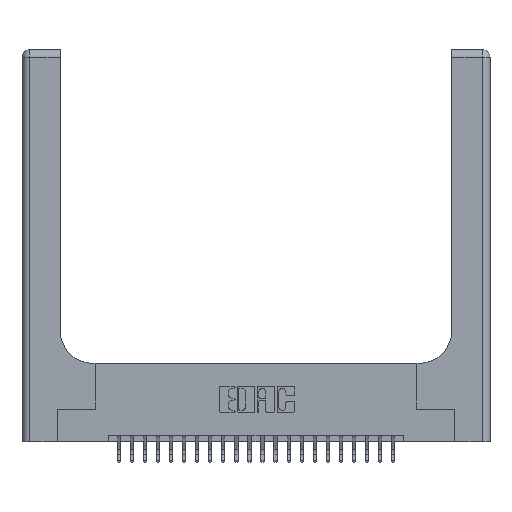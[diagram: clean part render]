
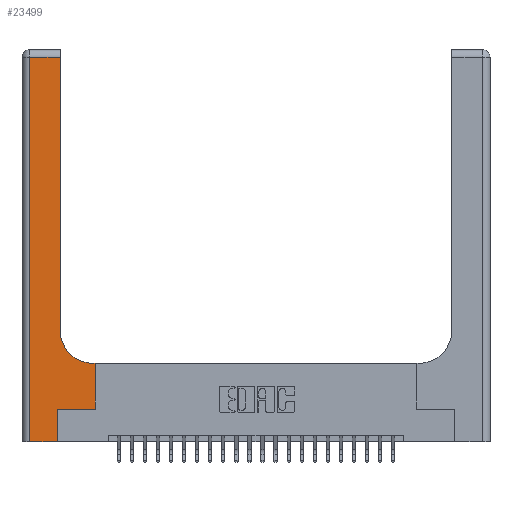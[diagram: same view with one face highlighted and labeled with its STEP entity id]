
A CAD part, top view. The second image highlights one B-rep face of the part: STEP entity #23499.
In plain terms, the highlighted planar face has unit normal (0, 0, 1).
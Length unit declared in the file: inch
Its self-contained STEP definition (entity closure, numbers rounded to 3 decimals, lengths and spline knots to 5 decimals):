
#33 = CARTESIAN_POINT ( 'NONE',  ( 0., 0., 0.37 ) ) ;
#120 = VECTOR ( 'NONE', #15755, 39.37008 ) ;
#164 = DIRECTION ( 'NONE',  ( 0., 1., 0. ) ) ;
#365 = LINE ( 'NONE', #9167, #15659 ) ;
#517 = CARTESIAN_POINT ( 'NONE',  ( 0.2915, 3., 0.37 ) ) ;
#683 = VERTEX_POINT ( 'NONE', #3446 ) ;
#2593 = EDGE_CURVE ( 'NONE', #6802, #8842, #365, .T. ) ;
#2601 = LINE ( 'NONE', #12190, #13845 ) ;
#2632 = EDGE_CURVE ( 'NONE', #4850, #683, #25175, .T. ) ;
#2824 = CARTESIAN_POINT ( 'NONE',  ( 0.269, 0., 0.37 ) ) ;
#3270 = DIRECTION ( 'NONE',  ( 0., 1., 0. ) ) ;
#3446 = CARTESIAN_POINT ( 'NONE',  ( 0.2915, 0.85, 0.37 ) ) ;
#4015 = ORIENTED_EDGE ( 'NONE', *, *, #16800, .T. ) ;
#4016 = EDGE_LOOP ( 'NONE', ( #20189, #21307, #7704, #24656, #18710, #25285, #23282, #4015, #7865 ) ) ;
#4236 = CARTESIAN_POINT ( 'NONE',  ( 0.269, 0.25, 0.37 ) ) ;
#4583 = DIRECTION ( 'NONE',  ( 0., 1., 0. ) ) ;
#4655 = LINE ( 'NONE', #24790, #24748 ) ;
#4850 = VERTEX_POINT ( 'NONE', #16974 ) ;
#5414 = VERTEX_POINT ( 'NONE', #6796 ) ;
#5592 = VERTEX_POINT ( 'NONE', #19182 ) ;
#5968 = EDGE_CURVE ( 'NONE', #683, #18829, #17972, .T. ) ;
#6436 = VECTOR ( 'NONE', #21737, 39.37008 ) ;
#6667 = VERTEX_POINT ( 'NONE', #16339 ) ;
#6796 = CARTESIAN_POINT ( 'NONE',  ( 0.06, 2.94, 0.37 ) ) ;
#6802 = VERTEX_POINT ( 'NONE', #2824 ) ;
#6946 = VECTOR ( 'NONE', #8156, 39.37008 ) ;
#7271 = CARTESIAN_POINT ( 'NONE',  ( 0.06, 3., 0.37 ) ) ;
#7704 = ORIENTED_EDGE ( 'NONE', *, *, #23745, .T. ) ;
#7865 = ORIENTED_EDGE ( 'NONE', *, *, #2632, .T. ) ;
#8156 = DIRECTION ( 'NONE',  ( 1., 0., 0. ) ) ;
#8186 = VECTOR ( 'NONE', #4583, 39.37008 ) ;
#8596 = DIRECTION ( 'NONE',  ( 0., 0., -1. ) ) ;
#8842 = VERTEX_POINT ( 'NONE', #4236 ) ;
#9167 = CARTESIAN_POINT ( 'NONE',  ( 0.269, 0., 0.37 ) ) ;
#9420 = DIRECTION ( 'NONE',  ( 0., 0., -1. ) ) ;
#9715 = AXIS2_PLACEMENT_3D ( 'NONE', #20992, #9420, #22915 ) ;
#10219 = CARTESIAN_POINT ( 'NONE',  ( 0.2915, 0.6, 0.37 ) ) ;
#10619 = VERTEX_POINT ( 'NONE', #14369 ) ;
#11457 = LINE ( 'NONE', #25306, #120 ) ;
#12158 = VECTOR ( 'NONE', #13254, 39.37008 ) ;
#12190 = CARTESIAN_POINT ( 'NONE',  ( 0.5585, 0.25, 0.37 ) ) ;
#12386 = LINE ( 'NONE', #10219, #6436 ) ;
#12619 = EDGE_CURVE ( 'NONE', #6667, #6802, #21847, .T. ) ;
#13254 = DIRECTION ( 'NONE',  ( 0., -1., 0. ) ) ;
#13845 = VECTOR ( 'NONE', #164, 39.37008 ) ;
#14369 = CARTESIAN_POINT ( 'NONE',  ( 0.5585, 0.6, 0.37 ) ) ;
#14398 = EDGE_CURVE ( 'NONE', #8842, #5592, #4655, .T. ) ;
#14405 = PLANE ( 'NONE',  #20089 ) ;
#15659 = VECTOR ( 'NONE', #3270, 39.37008 ) ;
#15755 = DIRECTION ( 'NONE',  ( -1., 0., 0. ) ) ;
#16339 = CARTESIAN_POINT ( 'NONE',  ( 0.06, 0., 0.37 ) ) ;
#16800 = EDGE_CURVE ( 'NONE', #10619, #4850, #12386, .T. ) ;
#16974 = CARTESIAN_POINT ( 'NONE',  ( 0.5415, 0.6, 0.37 ) ) ;
#17314 = LINE ( 'NONE', #7271, #12158 ) ;
#17972 = LINE ( 'NONE', #517, #8186 ) ;
#18207 = FACE_OUTER_BOUND ( 'NONE', #4016, .T. ) ;
#18710 = ORIENTED_EDGE ( 'NONE', *, *, #2593, .T. ) ;
#18829 = VERTEX_POINT ( 'NONE', #22611 ) ;
#19041 = DIRECTION ( 'NONE',  ( 1., 0., 0. ) ) ;
#19182 = CARTESIAN_POINT ( 'NONE',  ( 0.5585, 0.25, 0.37 ) ) ;
#20089 = AXIS2_PLACEMENT_3D ( 'NONE', #20214, #8596, #22118 ) ;
#20189 = ORIENTED_EDGE ( 'NONE', *, *, #5968, .T. ) ;
#20214 = CARTESIAN_POINT ( 'NONE',  ( 0., 3., 0.37 ) ) ;
#20545 = EDGE_CURVE ( 'NONE', #18829, #5414, #11457, .T. ) ;
#20992 = CARTESIAN_POINT ( 'NONE',  ( 0.5415, 0.85, 0.37 ) ) ;
#21307 = ORIENTED_EDGE ( 'NONE', *, *, #20545, .T. ) ;
#21737 = DIRECTION ( 'NONE',  ( -1., 0., 0. ) ) ;
#21792 = EDGE_CURVE ( 'NONE', #5592, #10619, #2601, .T. ) ;
#21847 = LINE ( 'NONE', #33, #6946 ) ;
#22118 = DIRECTION ( 'NONE',  ( -1., 0., 0. ) ) ;
#22611 = CARTESIAN_POINT ( 'NONE',  ( 0.2915, 2.94, 0.37 ) ) ;
#22915 = DIRECTION ( 'NONE',  ( 1., 0., 0. ) ) ;
#23282 = ORIENTED_EDGE ( 'NONE', *, *, #21792, .T. ) ;
#23499 = ADVANCED_FACE ( 'NONE', ( #18207 ), #14405, .F. ) ;
#23745 = EDGE_CURVE ( 'NONE', #5414, #6667, #17314, .T. ) ;
#24656 = ORIENTED_EDGE ( 'NONE', *, *, #12619, .T. ) ;
#24748 = VECTOR ( 'NONE', #19041, 39.37008 ) ;
#24790 = CARTESIAN_POINT ( 'NONE',  ( 0.269, 0.25, 0.37 ) ) ;
#25175 = CIRCLE ( 'NONE', #9715, 0.25 ) ;
#25285 = ORIENTED_EDGE ( 'NONE', *, *, #14398, .T. ) ;
#25306 = CARTESIAN_POINT ( 'NONE',  ( 0., 2.94, 0.37 ) ) ;
